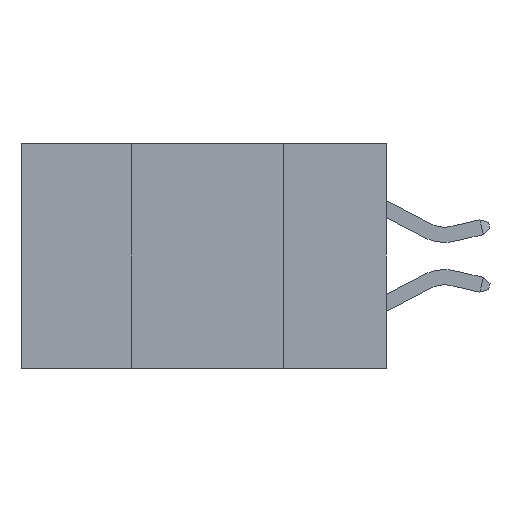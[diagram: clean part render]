
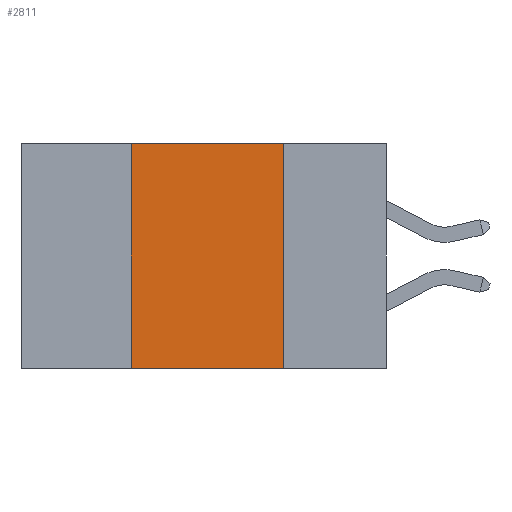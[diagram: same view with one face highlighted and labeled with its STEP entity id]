
A CAD part, left-side view. The second image highlights one B-rep face of the part: STEP entity #2811.
In plain terms, the highlighted planar face has unit normal (-1, 0, 0).
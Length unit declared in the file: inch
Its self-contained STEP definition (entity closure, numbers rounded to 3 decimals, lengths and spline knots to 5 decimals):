
#83 = CARTESIAN_POINT ( 'NONE',  ( 0., 0.42, 0. ) ) ;
#436 = DIRECTION ( 'NONE',  ( 0., 0., -1. ) ) ;
#852 = EDGE_CURVE ( 'NONE', #17856, #10477, #14921, .T. ) ;
#1173 = AXIS2_PLACEMENT_3D ( 'NONE', #15889, #3110, #436 ) ;
#2478 = VECTOR ( 'NONE', #19005, 39.37008 ) ;
#2811 = ADVANCED_FACE ( 'NONE', ( #13928 ), #3969, .F. ) ;
#3110 = DIRECTION ( 'NONE',  ( 1., 0., 0. ) ) ;
#3573 = VECTOR ( 'NONE', #8065, 39.37008 ) ;
#3969 = PLANE ( 'NONE',  #1173 ) ;
#4224 = CARTESIAN_POINT ( 'NONE',  ( 0., 0.17, -0.37 ) ) ;
#4784 = CARTESIAN_POINT ( 'NONE',  ( 0., 0.6, -0.37 ) ) ;
#4844 = DIRECTION ( 'NONE',  ( 0., -1., 0. ) ) ;
#5038 = EDGE_CURVE ( 'NONE', #10477, #15758, #6938, .T. ) ;
#5468 = ORIENTED_EDGE ( 'NONE', *, *, #14475, .T. ) ;
#5575 = VECTOR ( 'NONE', #17387, 39.37008 ) ;
#6938 = LINE ( 'NONE', #4224, #2478 ) ;
#8065 = DIRECTION ( 'NONE',  ( 0., -1., 0. ) ) ;
#8443 = VECTOR ( 'NONE', #4844, 39.37008 ) ;
#9345 = EDGE_LOOP ( 'NONE', ( #17929, #16561, #18158, #5468 ) ) ;
#10350 = VERTEX_POINT ( 'NONE', #11638 ) ;
#10477 = VERTEX_POINT ( 'NONE', #17774 ) ;
#10993 = EDGE_CURVE ( 'NONE', #10350, #17856, #12943, .T. ) ;
#11486 = CARTESIAN_POINT ( 'NONE',  ( 0., 0.42, -0.37 ) ) ;
#11638 = CARTESIAN_POINT ( 'NONE',  ( 0., 0.42, -0.37 ) ) ;
#12337 = CARTESIAN_POINT ( 'NONE',  ( 0., 0.6, 0. ) ) ;
#12943 = LINE ( 'NONE', #11486, #5575 ) ;
#13928 = FACE_OUTER_BOUND ( 'NONE', #9345, .T. ) ;
#14475 = EDGE_CURVE ( 'NONE', #10350, #15758, #16305, .T. ) ;
#14921 = LINE ( 'NONE', #12337, #3573 ) ;
#15758 = VERTEX_POINT ( 'NONE', #16437 ) ;
#15889 = CARTESIAN_POINT ( 'NONE',  ( 0., 0.6, 0. ) ) ;
#16305 = LINE ( 'NONE', #4784, #8443 ) ;
#16437 = CARTESIAN_POINT ( 'NONE',  ( 0., 0.17, -0.37 ) ) ;
#16561 = ORIENTED_EDGE ( 'NONE', *, *, #852, .F. ) ;
#17387 = DIRECTION ( 'NONE',  ( 0., 0., 1. ) ) ;
#17774 = CARTESIAN_POINT ( 'NONE',  ( 0., 0.17, 0. ) ) ;
#17856 = VERTEX_POINT ( 'NONE', #83 ) ;
#17929 = ORIENTED_EDGE ( 'NONE', *, *, #5038, .F. ) ;
#18158 = ORIENTED_EDGE ( 'NONE', *, *, #10993, .F. ) ;
#19005 = DIRECTION ( 'NONE',  ( 0., 0., -1. ) ) ;
